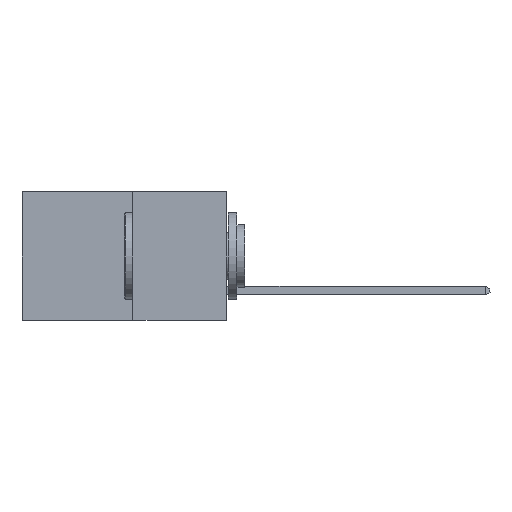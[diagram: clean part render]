
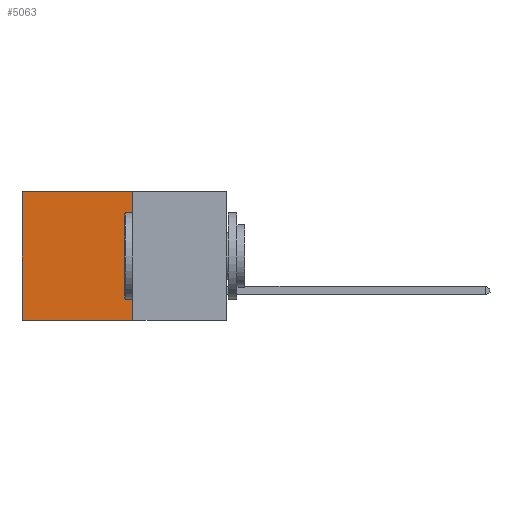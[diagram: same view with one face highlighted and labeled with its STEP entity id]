
A CAD part, left-side view. The second image highlights one B-rep face of the part: STEP entity #5063.
In plain terms, the highlighted planar face has unit normal (-1, 0, 0).
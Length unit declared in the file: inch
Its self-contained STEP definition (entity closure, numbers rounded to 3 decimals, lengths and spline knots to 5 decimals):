
#538 = EDGE_CURVE ( 'NONE', #8380, #4459, #10101, .T. ) ;
#767 = CARTESIAN_POINT ( 'NONE',  ( 0.277, 0.27, -0.37 ) ) ;
#815 = LINE ( 'NONE', #767, #12008 ) ;
#889 = EDGE_CURVE ( 'NONE', #4459, #4023, #7906, .T. ) ;
#971 = EDGE_CURVE ( 'NONE', #8380, #9046, #815, .T. ) ;
#1286 = DIRECTION ( 'NONE',  ( 0., 0., -1. ) ) ;
#2853 = DIRECTION ( 'NONE',  ( 0., 1., 0. ) ) ;
#3351 = ORIENTED_EDGE ( 'NONE', *, *, #889, .T. ) ;
#3373 = ORIENTED_EDGE ( 'NONE', *, *, #10168, .F. ) ;
#3438 = ORIENTED_EDGE ( 'NONE', *, *, #971, .F. ) ;
#3445 = CARTESIAN_POINT ( 'NONE',  ( 0.277, 0.59, -0.37 ) ) ;
#3456 = ORIENTED_EDGE ( 'NONE', *, *, #538, .T. ) ;
#4023 = VERTEX_POINT ( 'NONE', #13807 ) ;
#4082 = AXIS2_PLACEMENT_3D ( 'NONE', #13796, #8126, #1286 ) ;
#4459 = VERTEX_POINT ( 'NONE', #8617 ) ;
#4983 = PLANE ( 'NONE',  #4082 ) ;
#5063 = ADVANCED_FACE ( 'NONE', ( #6033 ), #4983, .F. ) ;
#6033 = FACE_OUTER_BOUND ( 'NONE', #6832, .T. ) ;
#6287 = CARTESIAN_POINT ( 'NONE',  ( 0.277, 0.27, -0.37 ) ) ;
#6832 = EDGE_LOOP ( 'NONE', ( #3351, #3373, #3438, #3456 ) ) ;
#7066 = DIRECTION ( 'NONE',  ( 0., 1., 0. ) ) ;
#7800 = VECTOR ( 'NONE', #7066, 39.37008 ) ;
#7834 = CARTESIAN_POINT ( 'NONE',  ( 0.277, 0.27, 0. ) ) ;
#7906 = LINE ( 'NONE', #3445, #9903 ) ;
#8126 = DIRECTION ( 'NONE',  ( 1., 0., 0. ) ) ;
#8380 = VERTEX_POINT ( 'NONE', #10159 ) ;
#8617 = CARTESIAN_POINT ( 'NONE',  ( 0.277, 0.59, 0. ) ) ;
#9046 = VERTEX_POINT ( 'NONE', #11951 ) ;
#9395 = DIRECTION ( 'NONE',  ( 0., 0., -1. ) ) ;
#9903 = VECTOR ( 'NONE', #9395, 39.37008 ) ;
#9968 = VECTOR ( 'NONE', #2853, 39.37008 ) ;
#10101 = LINE ( 'NONE', #7834, #7800 ) ;
#10159 = CARTESIAN_POINT ( 'NONE',  ( 0.277, 0.27, 0. ) ) ;
#10168 = EDGE_CURVE ( 'NONE', #9046, #4023, #12498, .T. ) ;
#10860 = DIRECTION ( 'NONE',  ( 0., 0., -1. ) ) ;
#11951 = CARTESIAN_POINT ( 'NONE',  ( 0.277, 0.27, -0.37 ) ) ;
#12008 = VECTOR ( 'NONE', #10860, 39.37008 ) ;
#12498 = LINE ( 'NONE', #6287, #9968 ) ;
#13796 = CARTESIAN_POINT ( 'NONE',  ( 0.277, 0.27, -0.37 ) ) ;
#13807 = CARTESIAN_POINT ( 'NONE',  ( 0.277, 0.59, -0.37 ) ) ;
